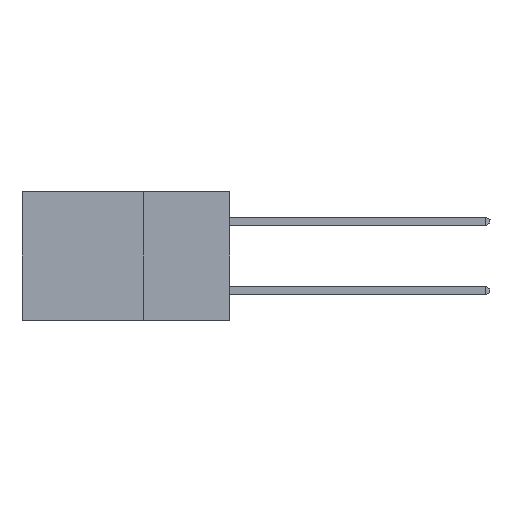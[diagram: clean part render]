
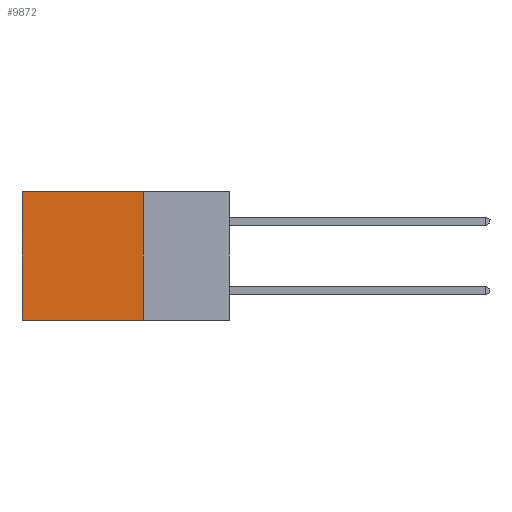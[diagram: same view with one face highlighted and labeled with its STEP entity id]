
A CAD part, left-side view. The second image highlights one B-rep face of the part: STEP entity #9872.
In plain terms, the highlighted planar face has unit normal (-1, 0, 0).
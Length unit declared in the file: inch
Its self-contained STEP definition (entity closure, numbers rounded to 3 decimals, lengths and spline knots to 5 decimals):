
#33 = CARTESIAN_POINT ( 'NONE',  ( 0.298, 0.25, 0. ) ) ;
#320 = LINE ( 'NONE', #20866, #13100 ) ;
#868 = DIRECTION ( 'NONE',  ( 0., 0., -1. ) ) ;
#2384 = VERTEX_POINT ( 'NONE', #20437 ) ;
#2939 = DIRECTION ( 'NONE',  ( 0., 1., 0. ) ) ;
#3952 = VERTEX_POINT ( 'NONE', #6537 ) ;
#5446 = CARTESIAN_POINT ( 'NONE',  ( 0.298, 0.6, 0. ) ) ;
#6537 = CARTESIAN_POINT ( 'NONE',  ( 0.298, 0.25, -0.37 ) ) ;
#7770 = CARTESIAN_POINT ( 'NONE',  ( 0.298, 0.25, 0. ) ) ;
#8520 = FACE_OUTER_BOUND ( 'NONE', #17773, .T. ) ;
#9312 = VECTOR ( 'NONE', #868, 39.37008 ) ;
#9596 = ORIENTED_EDGE ( 'NONE', *, *, #20952, .F. ) ;
#9719 = DIRECTION ( 'NONE',  ( 0., 0., -1. ) ) ;
#9872 = ADVANCED_FACE ( 'NONE', ( #8520 ), #13097, .F. ) ;
#10724 = VECTOR ( 'NONE', #14315, 39.37008 ) ;
#11323 = DIRECTION ( 'NONE',  ( 1., 0., 0. ) ) ;
#11927 = ORIENTED_EDGE ( 'NONE', *, *, #18217, .T. ) ;
#13097 = PLANE ( 'NONE',  #20777 ) ;
#13100 = VECTOR ( 'NONE', #17581, 39.37008 ) ;
#13148 = LINE ( 'NONE', #7770, #9312 ) ;
#14173 = VERTEX_POINT ( 'NONE', #33 ) ;
#14315 = DIRECTION ( 'NONE',  ( 0., 0., -1. ) ) ;
#14420 = LINE ( 'NONE', #17739, #10724 ) ;
#15068 = EDGE_CURVE ( 'NONE', #14173, #3952, #13148, .T. ) ;
#16037 = ORIENTED_EDGE ( 'NONE', *, *, #19057, .T. ) ;
#16270 = CARTESIAN_POINT ( 'NONE',  ( 0.298, 0.25, 0. ) ) ;
#16649 = ORIENTED_EDGE ( 'NONE', *, *, #15068, .F. ) ;
#17460 = LINE ( 'NONE', #17760, #18489 ) ;
#17581 = DIRECTION ( 'NONE',  ( 0., 1., 0. ) ) ;
#17739 = CARTESIAN_POINT ( 'NONE',  ( 0.298, 0.6, 0. ) ) ;
#17760 = CARTESIAN_POINT ( 'NONE',  ( 0.298, 0.25, 0. ) ) ;
#17773 = EDGE_LOOP ( 'NONE', ( #11927, #9596, #16649, #16037 ) ) ;
#18217 = EDGE_CURVE ( 'NONE', #18481, #2384, #14420, .T. ) ;
#18481 = VERTEX_POINT ( 'NONE', #5446 ) ;
#18489 = VECTOR ( 'NONE', #2939, 39.37008 ) ;
#19057 = EDGE_CURVE ( 'NONE', #14173, #18481, #17460, .T. ) ;
#20437 = CARTESIAN_POINT ( 'NONE',  ( 0.298, 0.6, -0.37 ) ) ;
#20777 = AXIS2_PLACEMENT_3D ( 'NONE', #16270, #11323, #9719 ) ;
#20866 = CARTESIAN_POINT ( 'NONE',  ( 0.298, 0.25, -0.37 ) ) ;
#20952 = EDGE_CURVE ( 'NONE', #3952, #2384, #320, .T. ) ;
